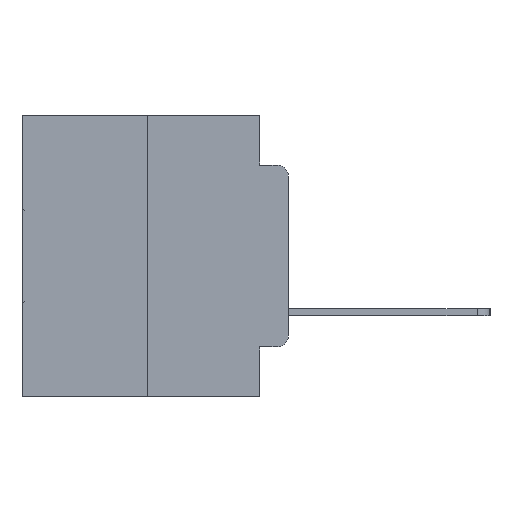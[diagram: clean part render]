
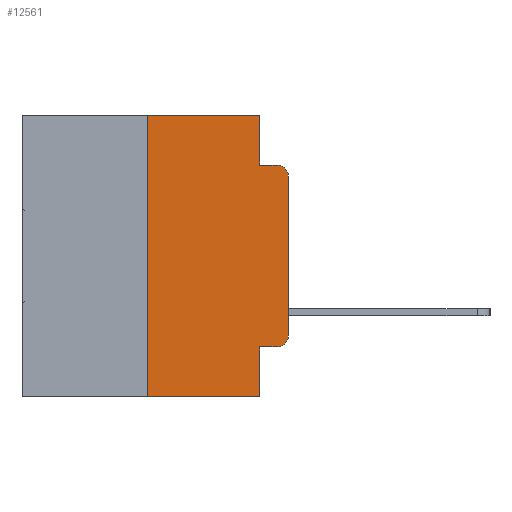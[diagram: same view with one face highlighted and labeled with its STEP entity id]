
A CAD part, left-side view. The second image highlights one B-rep face of the part: STEP entity #12561.
In plain terms, the highlighted planar face has unit normal (-1, 0, 0).
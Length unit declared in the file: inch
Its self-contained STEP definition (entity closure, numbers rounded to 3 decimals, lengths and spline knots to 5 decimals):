
#255 = CARTESIAN_POINT ( 'NONE',  ( 0., 0.02, -0.4115 ) ) ;
#806 = DIRECTION ( 'NONE',  ( 0., 0., -1. ) ) ;
#982 = LINE ( 'NONE', #12008, #1707 ) ;
#1678 = VERTEX_POINT ( 'NONE', #15098 ) ;
#1707 = VECTOR ( 'NONE', #27858, 39.37008 ) ;
#2006 = VERTEX_POINT ( 'NONE', #16596 ) ;
#2067 = ORIENTED_EDGE ( 'NONE', *, *, #16212, .F. ) ;
#2206 = FACE_OUTER_BOUND ( 'NONE', #10997, .T. ) ;
#3508 = DIRECTION ( 'NONE',  ( 0., 0., 1. ) ) ;
#3565 = ORIENTED_EDGE ( 'NONE', *, *, #7213, .T. ) ;
#3580 = DIRECTION ( 'NONE',  ( 0., -1., 0. ) ) ;
#3876 = VERTEX_POINT ( 'NONE', #26724 ) ;
#4080 = DIRECTION ( 'NONE',  ( 0., 0., -1. ) ) ;
#4091 = AXIS2_PLACEMENT_3D ( 'NONE', #14102, #29858, #16353 ) ;
#4468 = AXIS2_PLACEMENT_3D ( 'NONE', #7743, #23830, #10135 ) ;
#4645 = ORIENTED_EDGE ( 'NONE', *, *, #6798, .F. ) ;
#5251 = CIRCLE ( 'NONE', #4091, 0.02 ) ;
#5479 = EDGE_CURVE ( 'NONE', #1678, #25984, #982, .T. ) ;
#5521 = LINE ( 'NONE', #15269, #23211 ) ;
#5622 = VERTEX_POINT ( 'NONE', #12324 ) ;
#6599 = EDGE_CURVE ( 'NONE', #5622, #6833, #16661, .T. ) ;
#6798 = EDGE_CURVE ( 'NONE', #24902, #5622, #11644, .T. ) ;
#6833 = VERTEX_POINT ( 'NONE', #17535 ) ;
#6894 = VERTEX_POINT ( 'NONE', #15629 ) ;
#7213 = EDGE_CURVE ( 'NONE', #2006, #18876, #16987, .T. ) ;
#7556 = CARTESIAN_POINT ( 'NONE',  ( 0., 0., -0.1085 ) ) ;
#7743 = CARTESIAN_POINT ( 'NONE',  ( 0., 0.02, -0.3915 ) ) ;
#7838 = DIRECTION ( 'NONE',  ( 0., -1., 0. ) ) ;
#8169 = DIRECTION ( 'NONE',  ( 0., 0., -1. ) ) ;
#8395 = EDGE_CURVE ( 'NONE', #25984, #6833, #5251, .T. ) ;
#9753 = CARTESIAN_POINT ( 'NONE',  ( 0., 0.473, -0.5 ) ) ;
#9887 = EDGE_CURVE ( 'NONE', #6894, #24902, #5521, .T. ) ;
#10119 = CARTESIAN_POINT ( 'NONE',  ( 0., 0.051, -0.4115 ) ) ;
#10135 = DIRECTION ( 'NONE',  ( 0., 0., -1. ) ) ;
#10843 = VECTOR ( 'NONE', #7838, 39.37008 ) ;
#10997 = EDGE_LOOP ( 'NONE', ( #21662, #16350, #28396, #4645, #17796, #29773, #19899, #2067, #3565, #28032 ) ) ;
#11276 = VECTOR ( 'NONE', #14665, 39.37008 ) ;
#11460 = CIRCLE ( 'NONE', #4468, 0.02 ) ;
#11644 = LINE ( 'NONE', #24228, #29710 ) ;
#12008 = CARTESIAN_POINT ( 'NONE',  ( 0., 0., 0. ) ) ;
#12151 = VECTOR ( 'NONE', #3508, 39.37008 ) ;
#12324 = CARTESIAN_POINT ( 'NONE',  ( 0., 0.051, -0.0885 ) ) ;
#12561 = ADVANCED_FACE ( 'NONE', ( #2206 ), #28443, .F. ) ;
#14102 = CARTESIAN_POINT ( 'NONE',  ( 0., 0.02, -0.1085 ) ) ;
#14665 = DIRECTION ( 'NONE',  ( 0., -1., 0. ) ) ;
#15098 = CARTESIAN_POINT ( 'NONE',  ( 0., 0., -0.3915 ) ) ;
#15227 = CARTESIAN_POINT ( 'NONE',  ( 0., 0.051, 0. ) ) ;
#15269 = CARTESIAN_POINT ( 'NONE',  ( 0., 0.473, 0. ) ) ;
#15629 = CARTESIAN_POINT ( 'NONE',  ( 0., 0.25, 0. ) ) ;
#16212 = EDGE_CURVE ( 'NONE', #2006, #20311, #20473, .T. ) ;
#16350 = ORIENTED_EDGE ( 'NONE', *, *, #8395, .T. ) ;
#16353 = DIRECTION ( 'NONE',  ( 0., 0., -1. ) ) ;
#16596 = CARTESIAN_POINT ( 'NONE',  ( 0., 0.051, -0.4115 ) ) ;
#16661 = LINE ( 'NONE', #25922, #11276 ) ;
#16987 = LINE ( 'NONE', #10119, #10843 ) ;
#17367 = EDGE_CURVE ( 'NONE', #18876, #1678, #11460, .T. ) ;
#17535 = CARTESIAN_POINT ( 'NONE',  ( 0., 0.02, -0.0885 ) ) ;
#17796 = ORIENTED_EDGE ( 'NONE', *, *, #9887, .F. ) ;
#18228 = LINE ( 'NONE', #19758, #12151 ) ;
#18358 = EDGE_CURVE ( 'NONE', #3876, #6894, #18228, .T. ) ;
#18876 = VERTEX_POINT ( 'NONE', #255 ) ;
#19647 = CARTESIAN_POINT ( 'NONE',  ( 0., 0.051, -0.5 ) ) ;
#19758 = CARTESIAN_POINT ( 'NONE',  ( 0., 0.25, 0. ) ) ;
#19783 = VECTOR ( 'NONE', #4080, 39.37008 ) ;
#19899 = ORIENTED_EDGE ( 'NONE', *, *, #29670, .T. ) ;
#20311 = VERTEX_POINT ( 'NONE', #19647 ) ;
#20473 = LINE ( 'NONE', #24853, #19783 ) ;
#21662 = ORIENTED_EDGE ( 'NONE', *, *, #5479, .T. ) ;
#21919 = LINE ( 'NONE', #9753, #27198 ) ;
#23211 = VECTOR ( 'NONE', #3580, 39.37008 ) ;
#23367 = DIRECTION ( 'NONE',  ( 0., -1., 0. ) ) ;
#23830 = DIRECTION ( 'NONE',  ( -1., 0., 0. ) ) ;
#24228 = CARTESIAN_POINT ( 'NONE',  ( 0., 0.051, 0. ) ) ;
#24305 = AXIS2_PLACEMENT_3D ( 'NONE', #26159, #28354, #806 ) ;
#24853 = CARTESIAN_POINT ( 'NONE',  ( 0., 0.051, 0. ) ) ;
#24902 = VERTEX_POINT ( 'NONE', #15227 ) ;
#25922 = CARTESIAN_POINT ( 'NONE',  ( 0., 0.051, -0.0885 ) ) ;
#25984 = VERTEX_POINT ( 'NONE', #7556 ) ;
#26159 = CARTESIAN_POINT ( 'NONE',  ( 0., 0.473, 0. ) ) ;
#26724 = CARTESIAN_POINT ( 'NONE',  ( 0., 0.25, -0.5 ) ) ;
#27198 = VECTOR ( 'NONE', #23367, 39.37008 ) ;
#27858 = DIRECTION ( 'NONE',  ( 0., 0., 1. ) ) ;
#28032 = ORIENTED_EDGE ( 'NONE', *, *, #17367, .T. ) ;
#28354 = DIRECTION ( 'NONE',  ( 1., 0., 0. ) ) ;
#28396 = ORIENTED_EDGE ( 'NONE', *, *, #6599, .F. ) ;
#28443 = PLANE ( 'NONE',  #24305 ) ;
#29670 = EDGE_CURVE ( 'NONE', #3876, #20311, #21919, .T. ) ;
#29710 = VECTOR ( 'NONE', #8169, 39.37008 ) ;
#29773 = ORIENTED_EDGE ( 'NONE', *, *, #18358, .F. ) ;
#29858 = DIRECTION ( 'NONE',  ( -1., 0., 0. ) ) ;
